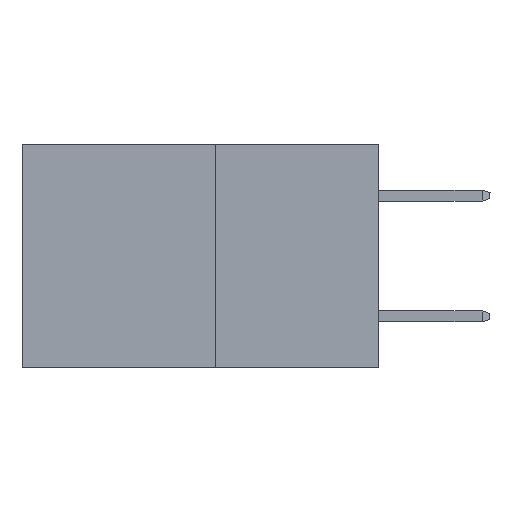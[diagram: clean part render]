
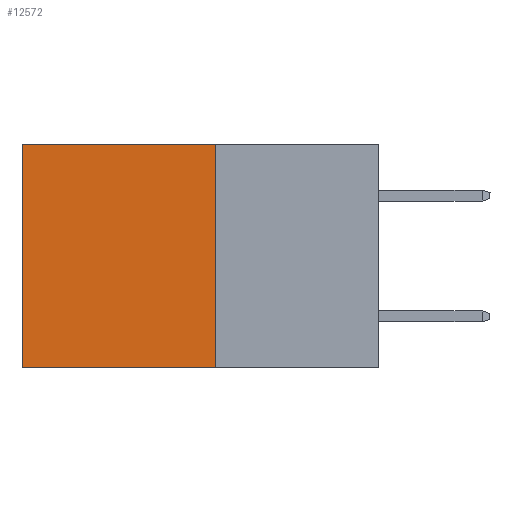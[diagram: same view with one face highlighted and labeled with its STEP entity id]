
A CAD part, left-side view. The second image highlights one B-rep face of the part: STEP entity #12572.
In plain terms, the highlighted planar face has unit normal (-1, 0, 0).
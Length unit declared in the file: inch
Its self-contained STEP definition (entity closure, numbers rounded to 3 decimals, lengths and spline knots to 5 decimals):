
#111 = DIRECTION ( 'NONE',  ( 0., 0., -1. ) ) ;
#264 = EDGE_CURVE ( 'NONE', #5359, #19767, #7552, .T. ) ;
#547 = PLANE ( 'NONE',  #16099 ) ;
#1140 = EDGE_CURVE ( 'NONE', #16672, #19767, #18479, .T. ) ;
#1999 = DIRECTION ( 'NONE',  ( 0., 1., 0. ) ) ;
#2179 = DIRECTION ( 'NONE',  ( 0., 0., -1. ) ) ;
#3654 = VECTOR ( 'NONE', #111, 39.37008 ) ;
#5359 = VERTEX_POINT ( 'NONE', #12856 ) ;
#5457 = EDGE_CURVE ( 'NONE', #20846, #5359, #16572, .T. ) ;
#6189 = VECTOR ( 'NONE', #10035, 39.37008 ) ;
#6330 = DIRECTION ( 'NONE',  ( 0., 1., 0. ) ) ;
#6732 = CARTESIAN_POINT ( 'NONE',  ( 0.277, 0.27, -0.37 ) ) ;
#6929 = EDGE_CURVE ( 'NONE', #20846, #16672, #12725, .T. ) ;
#7552 = LINE ( 'NONE', #6732, #11280 ) ;
#7622 = EDGE_LOOP ( 'NONE', ( #10191, #16233, #17974, #9000 ) ) ;
#7993 = CARTESIAN_POINT ( 'NONE',  ( 0.277, 0.27, 0. ) ) ;
#8525 = VECTOR ( 'NONE', #6330, 39.37008 ) ;
#9000 = ORIENTED_EDGE ( 'NONE', *, *, #6929, .T. ) ;
#9102 = CARTESIAN_POINT ( 'NONE',  ( 0.277, 0.59, -0.37 ) ) ;
#10035 = DIRECTION ( 'NONE',  ( 0., 0., -1. ) ) ;
#10191 = ORIENTED_EDGE ( 'NONE', *, *, #1140, .T. ) ;
#11280 = VECTOR ( 'NONE', #1999, 39.37008 ) ;
#11311 = CARTESIAN_POINT ( 'NONE',  ( 0.277, 0.59, -0.37 ) ) ;
#11987 = DIRECTION ( 'NONE',  ( 1., 0., 0. ) ) ;
#12572 = ADVANCED_FACE ( 'NONE', ( #18111 ), #547, .F. ) ;
#12725 = LINE ( 'NONE', #7993, #8525 ) ;
#12856 = CARTESIAN_POINT ( 'NONE',  ( 0.277, 0.27, -0.37 ) ) ;
#15762 = CARTESIAN_POINT ( 'NONE',  ( 0.277, 0.59, 0. ) ) ;
#16099 = AXIS2_PLACEMENT_3D ( 'NONE', #18388, #11987, #2179 ) ;
#16233 = ORIENTED_EDGE ( 'NONE', *, *, #264, .F. ) ;
#16449 = CARTESIAN_POINT ( 'NONE',  ( 0.277, 0.27, 0. ) ) ;
#16572 = LINE ( 'NONE', #19554, #3654 ) ;
#16672 = VERTEX_POINT ( 'NONE', #15762 ) ;
#17974 = ORIENTED_EDGE ( 'NONE', *, *, #5457, .F. ) ;
#18111 = FACE_OUTER_BOUND ( 'NONE', #7622, .T. ) ;
#18388 = CARTESIAN_POINT ( 'NONE',  ( 0.277, 0.27, -0.37 ) ) ;
#18479 = LINE ( 'NONE', #11311, #6189 ) ;
#19554 = CARTESIAN_POINT ( 'NONE',  ( 0.277, 0.27, -0.37 ) ) ;
#19767 = VERTEX_POINT ( 'NONE', #9102 ) ;
#20846 = VERTEX_POINT ( 'NONE', #16449 ) ;
